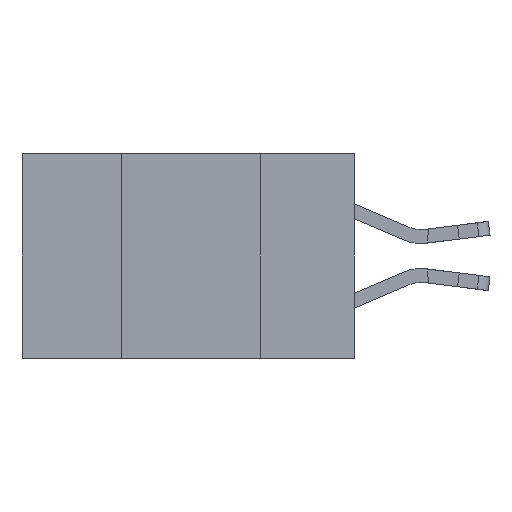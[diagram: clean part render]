
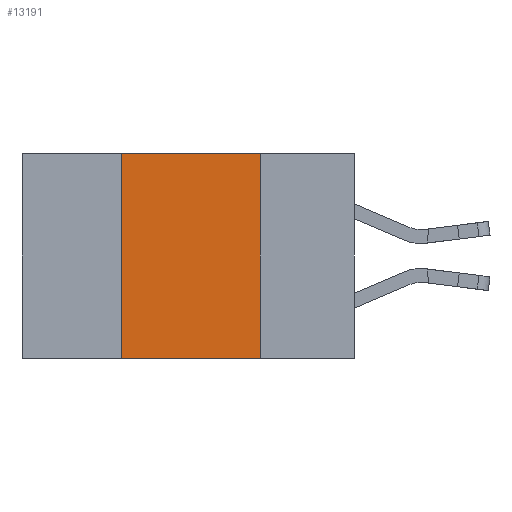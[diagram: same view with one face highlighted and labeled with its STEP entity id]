
A CAD part, left-side view. The second image highlights one B-rep face of the part: STEP entity #13191.
In plain terms, the highlighted planar face has unit normal (-1, 0, 0).
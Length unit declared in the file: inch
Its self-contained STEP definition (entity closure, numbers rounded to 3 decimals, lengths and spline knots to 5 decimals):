
#583 = DIRECTION ( 'NONE',  ( 0., -1., 0. ) ) ;
#1149 = VERTEX_POINT ( 'NONE', #14311 ) ;
#1950 = LINE ( 'NONE', #5107, #14011 ) ;
#2430 = DIRECTION ( 'NONE',  ( 1., 0., 0. ) ) ;
#2635 = LINE ( 'NONE', #15468, #15817 ) ;
#2714 = ORIENTED_EDGE ( 'NONE', *, *, #15230, .F. ) ;
#2721 = FACE_OUTER_BOUND ( 'NONE', #10021, .T. ) ;
#2738 = CARTESIAN_POINT ( 'NONE',  ( 0., 0.17, -0.37 ) ) ;
#3124 = ORIENTED_EDGE ( 'NONE', *, *, #6797, .F. ) ;
#3889 = DIRECTION ( 'NONE',  ( 0., 0., -1. ) ) ;
#5107 = CARTESIAN_POINT ( 'NONE',  ( 0., 0.17, 0. ) ) ;
#5605 = CARTESIAN_POINT ( 'NONE',  ( 0., 0.42, 0. ) ) ;
#5960 = EDGE_CURVE ( 'NONE', #13669, #10954, #1950, .T. ) ;
#6299 = CARTESIAN_POINT ( 'NONE',  ( 0., 0.42, 0. ) ) ;
#6480 = ORIENTED_EDGE ( 'NONE', *, *, #7618, .T. ) ;
#6655 = LINE ( 'NONE', #15922, #16061 ) ;
#6797 = EDGE_CURVE ( 'NONE', #1149, #13890, #11327, .T. ) ;
#7122 = CARTESIAN_POINT ( 'NONE',  ( 0., 0.17, 0. ) ) ;
#7618 = EDGE_CURVE ( 'NONE', #1149, #10954, #6655, .T. ) ;
#8678 = PLANE ( 'NONE',  #13141 ) ;
#9953 = CARTESIAN_POINT ( 'NONE',  ( 0., 0.6, 0. ) ) ;
#10021 = EDGE_LOOP ( 'NONE', ( #15505, #2714, #3124, #6480 ) ) ;
#10618 = DIRECTION ( 'NONE',  ( 0., 0., 1. ) ) ;
#10954 = VERTEX_POINT ( 'NONE', #2738 ) ;
#11177 = DIRECTION ( 'NONE',  ( 0., 0., -1. ) ) ;
#11327 = LINE ( 'NONE', #5605, #14588 ) ;
#12326 = DIRECTION ( 'NONE',  ( 0., -1., 0. ) ) ;
#13141 = AXIS2_PLACEMENT_3D ( 'NONE', #9953, #2430, #11177 ) ;
#13191 = ADVANCED_FACE ( 'NONE', ( #2721 ), #8678, .F. ) ;
#13669 = VERTEX_POINT ( 'NONE', #7122 ) ;
#13890 = VERTEX_POINT ( 'NONE', #6299 ) ;
#14011 = VECTOR ( 'NONE', #3889, 39.37008 ) ;
#14311 = CARTESIAN_POINT ( 'NONE',  ( 0., 0.42, -0.37 ) ) ;
#14588 = VECTOR ( 'NONE', #10618, 39.37008 ) ;
#15230 = EDGE_CURVE ( 'NONE', #13890, #13669, #2635, .T. ) ;
#15468 = CARTESIAN_POINT ( 'NONE',  ( 0., 0.6, 0. ) ) ;
#15505 = ORIENTED_EDGE ( 'NONE', *, *, #5960, .F. ) ;
#15817 = VECTOR ( 'NONE', #583, 39.37008 ) ;
#15922 = CARTESIAN_POINT ( 'NONE',  ( 0., 0.6, -0.37 ) ) ;
#16061 = VECTOR ( 'NONE', #12326, 39.37008 ) ;
